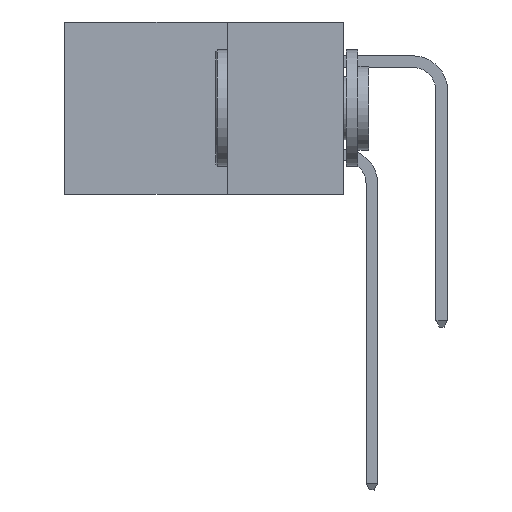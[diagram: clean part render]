
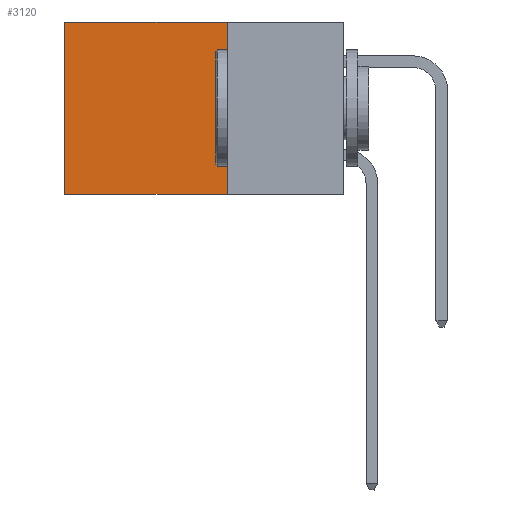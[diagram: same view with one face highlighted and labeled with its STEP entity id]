
A CAD part, left-side view. The second image highlights one B-rep face of the part: STEP entity #3120.
In plain terms, the highlighted planar face has unit normal (-1, 0, 0).
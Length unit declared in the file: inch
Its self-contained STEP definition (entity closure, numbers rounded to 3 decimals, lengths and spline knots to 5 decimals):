
#454 = LINE ( 'NONE', #4725, #9100 ) ;
#1451 = EDGE_CURVE ( 'NONE', #4460, #9278, #4183, .T. ) ;
#1482 = PLANE ( 'NONE',  #3477 ) ;
#2193 = DIRECTION ( 'NONE',  ( 1., 0., 0. ) ) ;
#2617 = DIRECTION ( 'NONE',  ( 0., 0., -1. ) ) ;
#2663 = EDGE_CURVE ( 'NONE', #5418, #4460, #9979, .T. ) ;
#3045 = DIRECTION ( 'NONE',  ( 0., 1., 0. ) ) ;
#3120 = ADVANCED_FACE ( 'NONE', ( #10827 ), #1482, .F. ) ;
#3477 = AXIS2_PLACEMENT_3D ( 'NONE', #4814, #2193, #7374 ) ;
#4146 = CARTESIAN_POINT ( 'NONE',  ( 0.2615, 0.6, 0. ) ) ;
#4183 = LINE ( 'NONE', #7590, #8222 ) ;
#4460 = VERTEX_POINT ( 'NONE', #4146 ) ;
#4638 = ORIENTED_EDGE ( 'NONE', *, *, #8738, .F. ) ;
#4725 = CARTESIAN_POINT ( 'NONE',  ( 0.2615, 0.25, -0.37 ) ) ;
#4814 = CARTESIAN_POINT ( 'NONE',  ( 0.2615, 0.25, -0.37 ) ) ;
#5008 = CARTESIAN_POINT ( 'NONE',  ( 0.2615, 0.25, -0.37 ) ) ;
#5127 = EDGE_LOOP ( 'NONE', ( #7266, #10922, #4638, #10727 ) ) ;
#5418 = VERTEX_POINT ( 'NONE', #6574 ) ;
#5682 = EDGE_CURVE ( 'NONE', #5908, #9278, #454, .T. ) ;
#5908 = VERTEX_POINT ( 'NONE', #6821 ) ;
#6574 = CARTESIAN_POINT ( 'NONE',  ( 0.2615, 0.25, 0. ) ) ;
#6779 = VECTOR ( 'NONE', #10947, 39.37008 ) ;
#6821 = CARTESIAN_POINT ( 'NONE',  ( 0.2615, 0.25, -0.37 ) ) ;
#7266 = ORIENTED_EDGE ( 'NONE', *, *, #1451, .T. ) ;
#7374 = DIRECTION ( 'NONE',  ( 0., 0., -1. ) ) ;
#7503 = LINE ( 'NONE', #5008, #6779 ) ;
#7590 = CARTESIAN_POINT ( 'NONE',  ( 0.2615, 0.6, -0.37 ) ) ;
#8222 = VECTOR ( 'NONE', #2617, 39.37008 ) ;
#8335 = VECTOR ( 'NONE', #9154, 39.37008 ) ;
#8569 = CARTESIAN_POINT ( 'NONE',  ( 0.2615, 0.6, -0.37 ) ) ;
#8738 = EDGE_CURVE ( 'NONE', #5418, #5908, #7503, .T. ) ;
#9100 = VECTOR ( 'NONE', #3045, 39.37008 ) ;
#9154 = DIRECTION ( 'NONE',  ( 0., 1., 0. ) ) ;
#9278 = VERTEX_POINT ( 'NONE', #8569 ) ;
#9979 = LINE ( 'NONE', #10802, #8335 ) ;
#10727 = ORIENTED_EDGE ( 'NONE', *, *, #2663, .T. ) ;
#10802 = CARTESIAN_POINT ( 'NONE',  ( 0.2615, 0.25, 0. ) ) ;
#10827 = FACE_OUTER_BOUND ( 'NONE', #5127, .T. ) ;
#10922 = ORIENTED_EDGE ( 'NONE', *, *, #5682, .F. ) ;
#10947 = DIRECTION ( 'NONE',  ( 0., 0., -1. ) ) ;
